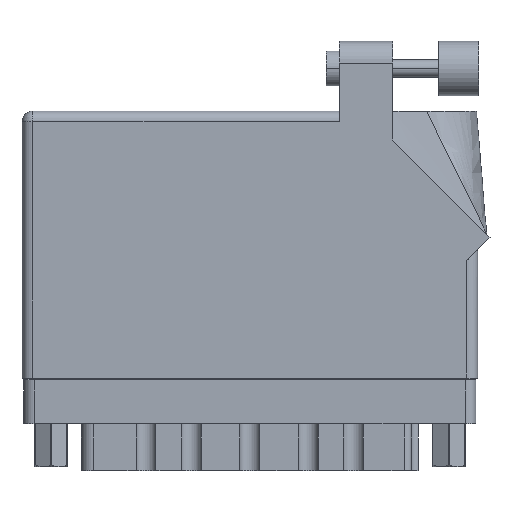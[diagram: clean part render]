
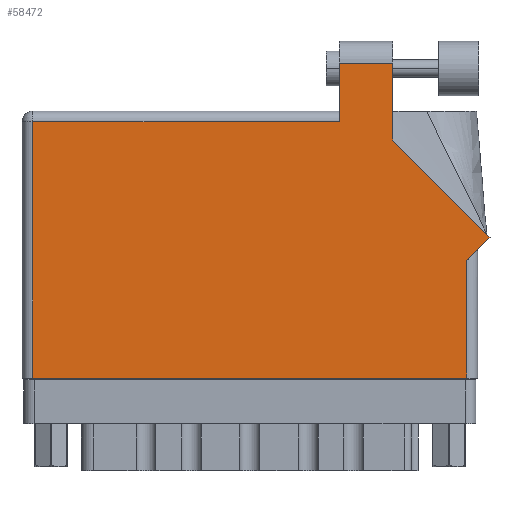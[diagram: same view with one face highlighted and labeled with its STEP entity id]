
A CAD part, front view. The second image highlights one B-rep face of the part: STEP entity #58472.
In plain terms, the highlighted face is planar.
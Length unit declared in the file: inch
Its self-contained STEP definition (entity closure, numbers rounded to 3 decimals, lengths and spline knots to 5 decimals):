
#1178 = DIRECTION ( 'NONE',  ( 0., 1., 0. ) ) ;
#1802 = CARTESIAN_POINT ( 'NONE',  ( 2.55, 0.675, 0. ) ) ;
#3445 = CARTESIAN_POINT ( 'NONE',  ( 2.126, 1.36442, 0. ) ) ;
#3660 = FACE_OUTER_BOUND ( 'NONE', #22392, .T. ) ;
#3665 = DIRECTION ( 'NONE',  ( 0., -1., 0. ) ) ;
#3776 = VECTOR ( 'NONE', #3665, 39.37008 ) ;
#4399 = DIRECTION ( 'NONE',  ( 0., 0., -1. ) ) ;
#4457 = DIRECTION ( 'NONE',  ( -1., 0., 0. ) ) ;
#4631 = AXIS2_PLACEMENT_3D ( 'NONE', #45167, #4399, #19534 ) ;
#4918 = EDGE_CURVE ( 'NONE', #61746, #13664, #43948, .T. ) ;
#5538 = ORIENTED_EDGE ( 'NONE', *, *, #31749, .T. ) ;
#5592 = VECTOR ( 'NONE', #20355, 39.37008 ) ;
#5626 = ORIENTED_EDGE ( 'NONE', *, *, #15197, .T. ) ;
#6420 = CARTESIAN_POINT ( 'NONE',  ( 2.55, 0., 0. ) ) ;
#6676 = CARTESIAN_POINT ( 'NONE',  ( 2.126, 1.805, 0. ) ) ;
#6710 = PLANE ( 'NONE',  #4631 ) ;
#6763 = LINE ( 'NONE', #42560, #3776 ) ;
#7361 = EDGE_CURVE ( 'NONE', #40487, #26331, #38277, .T. ) ;
#8884 = DIRECTION ( 'NONE',  ( -0.707, 0.707, 0. ) ) ;
#10419 = VECTOR ( 'NONE', #1178, 39.37008 ) ;
#11224 = VECTOR ( 'NONE', #41712, 39.37008 ) ;
#11418 = CARTESIAN_POINT ( 'NONE',  ( 1.819, 1.468, 0. ) ) ;
#12057 = LINE ( 'NONE', #13324, #30908 ) ;
#12482 = CARTESIAN_POINT ( 'NONE',  ( 0.062, 0., 0. ) ) ;
#13077 = LINE ( 'NONE', #12482, #51345 ) ;
#13324 = CARTESIAN_POINT ( 'NONE',  ( 2.68271, 0.80771, 0. ) ) ;
#13664 = VERTEX_POINT ( 'NONE', #47116 ) ;
#14891 = ORIENTED_EDGE ( 'NONE', *, *, #4918, .T. ) ;
#15162 = VERTEX_POINT ( 'NONE', #3445 ) ;
#15197 = EDGE_CURVE ( 'NONE', #26331, #19583, #25638, .T. ) ;
#15707 = ORIENTED_EDGE ( 'NONE', *, *, #26291, .T. ) ;
#15986 = VERTEX_POINT ( 'NONE', #29079 ) ;
#17179 = ORIENTED_EDGE ( 'NONE', *, *, #29336, .T. ) ;
#19534 = DIRECTION ( 'NONE',  ( -1., 0., 0. ) ) ;
#19583 = VERTEX_POINT ( 'NONE', #26751 ) ;
#20355 = DIRECTION ( 'NONE',  ( -1., 0., 0. ) ) ;
#20798 = VERTEX_POINT ( 'NONE', #43546 ) ;
#22392 = EDGE_LOOP ( 'NONE', ( #30486, #14891, #42842, #5538, #15707, #61398, #27165, #5626, #17179 ) ) ;
#23708 = CARTESIAN_POINT ( 'NONE',  ( 2.126, 1.36442, 0. ) ) ;
#25235 = LINE ( 'NONE', #62016, #44718 ) ;
#25638 = LINE ( 'NONE', #56161, #11224 ) ;
#26232 = VERTEX_POINT ( 'NONE', #11418 ) ;
#26291 = EDGE_CURVE ( 'NONE', #20798, #15986, #13077, .T. ) ;
#26331 = VERTEX_POINT ( 'NONE', #1802 ) ;
#26751 = CARTESIAN_POINT ( 'NONE',  ( 2.68271, 0.80771, 0. ) ) ;
#27165 = ORIENTED_EDGE ( 'NONE', *, *, #7361, .T. ) ;
#29079 = CARTESIAN_POINT ( 'NONE',  ( 0.062, 0., 0. ) ) ;
#29336 = EDGE_CURVE ( 'NONE', #19583, #15162, #12057, .T. ) ;
#30486 = ORIENTED_EDGE ( 'NONE', *, *, #30814, .T. ) ;
#30814 = EDGE_CURVE ( 'NONE', #15162, #61746, #50911, .T. ) ;
#30908 = VECTOR ( 'NONE', #8884, 39.37008 ) ;
#31749 = EDGE_CURVE ( 'NONE', #26232, #20798, #25235, .T. ) ;
#32238 = VECTOR ( 'NONE', #38913, 39.37008 ) ;
#35492 = CARTESIAN_POINT ( 'NONE',  ( 1.819, 1.805, 0. ) ) ;
#38277 = LINE ( 'NONE', #58739, #10419 ) ;
#38913 = DIRECTION ( 'NONE',  ( 1., 0., 0. ) ) ;
#40487 = VERTEX_POINT ( 'NONE', #6420 ) ;
#41674 = EDGE_CURVE ( 'NONE', #15986, #40487, #60025, .T. ) ;
#41712 = DIRECTION ( 'NONE',  ( 0.707, 0.707, 0. ) ) ;
#42560 = CARTESIAN_POINT ( 'NONE',  ( 1.819, 1.53, 0. ) ) ;
#42842 = ORIENTED_EDGE ( 'NONE', *, *, #47658, .T. ) ;
#43546 = CARTESIAN_POINT ( 'NONE',  ( 0.062, 1.468, 0. ) ) ;
#43948 = LINE ( 'NONE', #35492, #5592 ) ;
#44718 = VECTOR ( 'NONE', #4457, 39.37008 ) ;
#45167 = CARTESIAN_POINT ( 'NONE',  ( 0., 1.53, 0. ) ) ;
#47116 = CARTESIAN_POINT ( 'NONE',  ( 1.819, 1.805, 0. ) ) ;
#47658 = EDGE_CURVE ( 'NONE', #13664, #26232, #6763, .T. ) ;
#49415 = VECTOR ( 'NONE', #53230, 39.37008 ) ;
#50627 = DIRECTION ( 'NONE',  ( 0., -1., 0. ) ) ;
#50911 = LINE ( 'NONE', #23708, #49415 ) ;
#51345 = VECTOR ( 'NONE', #50627, 39.37008 ) ;
#53230 = DIRECTION ( 'NONE',  ( 0., 1., 0. ) ) ;
#56161 = CARTESIAN_POINT ( 'NONE',  ( 2.612, 0.737, 0. ) ) ;
#57976 = CARTESIAN_POINT ( 'NONE',  ( 0., 0., 0. ) ) ;
#58472 = ADVANCED_FACE ( 'NONE', ( #3660 ), #6710, .F. ) ;
#58739 = CARTESIAN_POINT ( 'NONE',  ( 2.55, 0.737, 0. ) ) ;
#60025 = LINE ( 'NONE', #57976, #32238 ) ;
#61398 = ORIENTED_EDGE ( 'NONE', *, *, #41674, .T. ) ;
#61746 = VERTEX_POINT ( 'NONE', #6676 ) ;
#62016 = CARTESIAN_POINT ( 'NONE',  ( 0., 1.468, 0. ) ) ;
